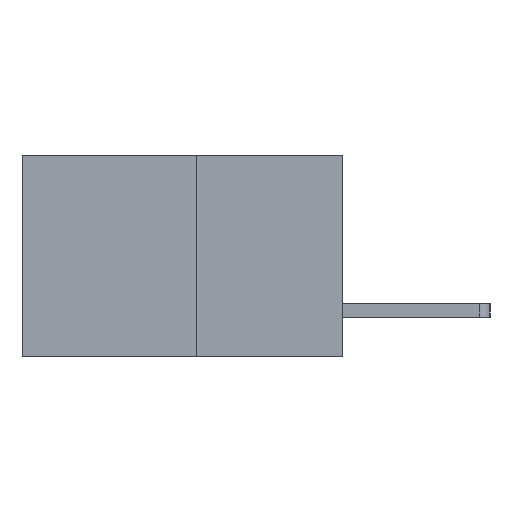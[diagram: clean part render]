
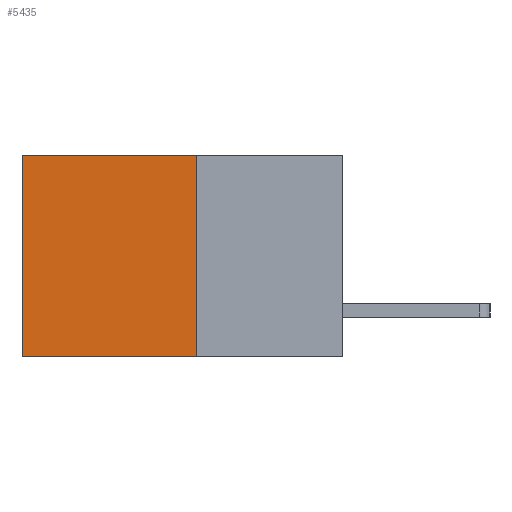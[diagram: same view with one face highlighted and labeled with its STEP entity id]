
A CAD part, left-side view. The second image highlights one B-rep face of the part: STEP entity #5435.
In plain terms, the highlighted planar face has unit normal (-1, 0, 0).
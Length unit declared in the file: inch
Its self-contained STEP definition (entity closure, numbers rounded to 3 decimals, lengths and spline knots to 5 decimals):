
#824 = EDGE_CURVE ( 'NONE', #3489, #2156, #5953, .T. ) ;
#1900 = DIRECTION ( 'NONE',  ( 0., 1., 0. ) ) ;
#1910 = CARTESIAN_POINT ( 'NONE',  ( 0.277, 0.27, -0.37 ) ) ;
#1987 = DIRECTION ( 'NONE',  ( 0., 1., 0. ) ) ;
#2115 = CARTESIAN_POINT ( 'NONE',  ( 0.277, 0.27, -0.37 ) ) ;
#2154 = CARTESIAN_POINT ( 'NONE',  ( 0.277, 0.59, 0. ) ) ;
#2156 = VERTEX_POINT ( 'NONE', #9744 ) ;
#2793 = ORIENTED_EDGE ( 'NONE', *, *, #824, .F. ) ;
#2796 = EDGE_CURVE ( 'NONE', #2156, #5432, #10110, .T. ) ;
#3069 = LINE ( 'NONE', #8805, #5148 ) ;
#3489 = VERTEX_POINT ( 'NONE', #9346 ) ;
#3607 = PLANE ( 'NONE',  #7140 ) ;
#3965 = CARTESIAN_POINT ( 'NONE',  ( 0.277, 0.59, -0.37 ) ) ;
#4242 = VECTOR ( 'NONE', #9860, 39.37008 ) ;
#4477 = DIRECTION ( 'NONE',  ( 1., 0., 0. ) ) ;
#5148 = VECTOR ( 'NONE', #1900, 39.37008 ) ;
#5432 = VERTEX_POINT ( 'NONE', #7842 ) ;
#5435 = ADVANCED_FACE ( 'NONE', ( #10051 ), #3607, .F. ) ;
#5953 = LINE ( 'NONE', #1910, #10411 ) ;
#6252 = ORIENTED_EDGE ( 'NONE', *, *, #7114, .T. ) ;
#7114 = EDGE_CURVE ( 'NONE', #10515, #5432, #8980, .T. ) ;
#7140 = AXIS2_PLACEMENT_3D ( 'NONE', #9493, #4477, #10358 ) ;
#7401 = DIRECTION ( 'NONE',  ( 0., 0., -1. ) ) ;
#7442 = EDGE_LOOP ( 'NONE', ( #6252, #9510, #2793, #8116 ) ) ;
#7842 = CARTESIAN_POINT ( 'NONE',  ( 0.277, 0.59, -0.37 ) ) ;
#8116 = ORIENTED_EDGE ( 'NONE', *, *, #9140, .T. ) ;
#8805 = CARTESIAN_POINT ( 'NONE',  ( 0.277, 0.27, 0. ) ) ;
#8980 = LINE ( 'NONE', #3965, #4242 ) ;
#9140 = EDGE_CURVE ( 'NONE', #3489, #10515, #3069, .T. ) ;
#9346 = CARTESIAN_POINT ( 'NONE',  ( 0.277, 0.27, 0. ) ) ;
#9493 = CARTESIAN_POINT ( 'NONE',  ( 0.277, 0.27, -0.37 ) ) ;
#9510 = ORIENTED_EDGE ( 'NONE', *, *, #2796, .F. ) ;
#9744 = CARTESIAN_POINT ( 'NONE',  ( 0.277, 0.27, -0.37 ) ) ;
#9860 = DIRECTION ( 'NONE',  ( 0., 0., -1. ) ) ;
#10051 = FACE_OUTER_BOUND ( 'NONE', #7442, .T. ) ;
#10110 = LINE ( 'NONE', #2115, #10374 ) ;
#10358 = DIRECTION ( 'NONE',  ( 0., 0., -1. ) ) ;
#10374 = VECTOR ( 'NONE', #1987, 39.37008 ) ;
#10411 = VECTOR ( 'NONE', #7401, 39.37008 ) ;
#10515 = VERTEX_POINT ( 'NONE', #2154 ) ;
